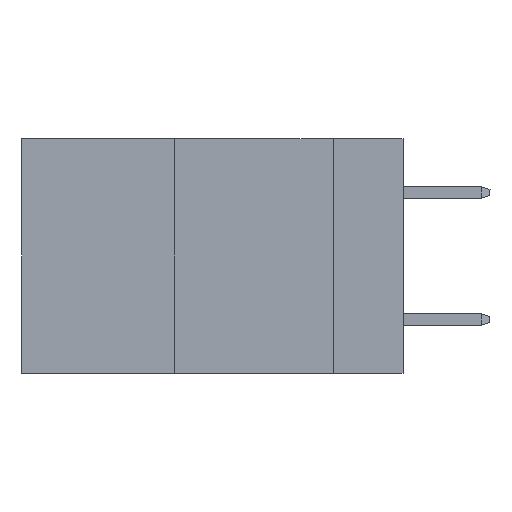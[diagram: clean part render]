
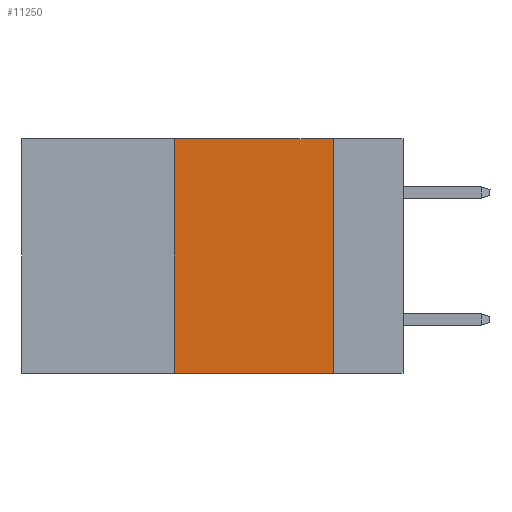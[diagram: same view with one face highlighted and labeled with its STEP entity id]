
A CAD part, left-side view. The second image highlights one B-rep face of the part: STEP entity #11250.
In plain terms, the highlighted planar face has unit normal (-1, 0, 0).
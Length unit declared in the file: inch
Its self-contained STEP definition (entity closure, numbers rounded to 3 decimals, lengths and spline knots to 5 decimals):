
#143 = EDGE_CURVE ( 'NONE', #2855, #15537, #8162, .T. ) ;
#241 = CARTESIAN_POINT ( 'NONE',  ( 0., 0.36, 0. ) ) ;
#723 = ORIENTED_EDGE ( 'NONE', *, *, #143, .T. ) ;
#771 = CARTESIAN_POINT ( 'NONE',  ( 0., 0.11, -0.37 ) ) ;
#914 = DIRECTION ( 'NONE',  ( 0., 0., -1. ) ) ;
#1029 = AXIS2_PLACEMENT_3D ( 'NONE', #9777, #14987, #3325 ) ;
#2061 = EDGE_LOOP ( 'NONE', ( #14837, #16189, #10887, #723 ) ) ;
#2855 = VERTEX_POINT ( 'NONE', #3868 ) ;
#3325 = DIRECTION ( 'NONE',  ( 0., 0., -1. ) ) ;
#3868 = CARTESIAN_POINT ( 'NONE',  ( 0., 0.36, -0.37 ) ) ;
#4613 = PLANE ( 'NONE',  #1029 ) ;
#4644 = DIRECTION ( 'NONE',  ( 0., -1., 0. ) ) ;
#5550 = CARTESIAN_POINT ( 'NONE',  ( 0., 0.6, -0.37 ) ) ;
#6138 = VECTOR ( 'NONE', #14915, 39.37008 ) ;
#6269 = CARTESIAN_POINT ( 'NONE',  ( 0., 0.11, 0. ) ) ;
#6673 = VECTOR ( 'NONE', #13078, 39.37008 ) ;
#6792 = VECTOR ( 'NONE', #914, 39.37008 ) ;
#7316 = VERTEX_POINT ( 'NONE', #241 ) ;
#7568 = EDGE_CURVE ( 'NONE', #2855, #7316, #14376, .T. ) ;
#8162 = LINE ( 'NONE', #5550, #6138 ) ;
#9483 = CARTESIAN_POINT ( 'NONE',  ( 0., 0.11, 0. ) ) ;
#9635 = LINE ( 'NONE', #13401, #11771 ) ;
#9777 = CARTESIAN_POINT ( 'NONE',  ( 0., 0.6, 0. ) ) ;
#10887 = ORIENTED_EDGE ( 'NONE', *, *, #7568, .F. ) ;
#11065 = FACE_OUTER_BOUND ( 'NONE', #2061, .T. ) ;
#11250 = ADVANCED_FACE ( 'NONE', ( #11065 ), #4613, .F. ) ;
#11771 = VECTOR ( 'NONE', #4644, 39.37008 ) ;
#12557 = LINE ( 'NONE', #6269, #6792 ) ;
#13078 = DIRECTION ( 'NONE',  ( 0., 0., 1. ) ) ;
#13401 = CARTESIAN_POINT ( 'NONE',  ( 0., 0.6, 0. ) ) ;
#13504 = EDGE_CURVE ( 'NONE', #15828, #15537, #12557, .T. ) ;
#14376 = LINE ( 'NONE', #15485, #6673 ) ;
#14837 = ORIENTED_EDGE ( 'NONE', *, *, #13504, .F. ) ;
#14915 = DIRECTION ( 'NONE',  ( 0., -1., 0. ) ) ;
#14987 = DIRECTION ( 'NONE',  ( 1., 0., 0. ) ) ;
#15485 = CARTESIAN_POINT ( 'NONE',  ( 0., 0.36, 0. ) ) ;
#15537 = VERTEX_POINT ( 'NONE', #771 ) ;
#15828 = VERTEX_POINT ( 'NONE', #9483 ) ;
#16189 = ORIENTED_EDGE ( 'NONE', *, *, #16426, .F. ) ;
#16426 = EDGE_CURVE ( 'NONE', #7316, #15828, #9635, .T. ) ;
